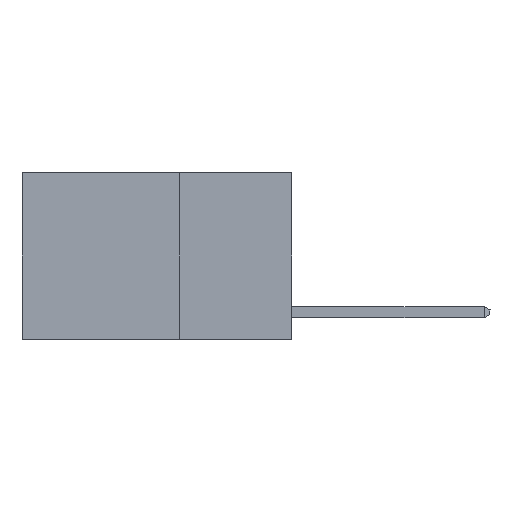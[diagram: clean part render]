
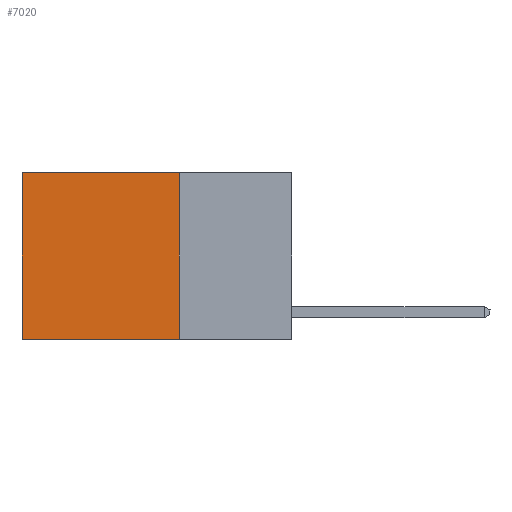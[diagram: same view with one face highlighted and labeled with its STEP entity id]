
A CAD part, left-side view. The second image highlights one B-rep face of the part: STEP entity #7020.
In plain terms, the highlighted planar face has unit normal (-1, 0, 0).
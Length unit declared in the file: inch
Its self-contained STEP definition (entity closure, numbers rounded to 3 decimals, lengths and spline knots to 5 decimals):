
#259 = LINE ( 'NONE', #1123, #986 ) ;
#496 = ORIENTED_EDGE ( 'NONE', *, *, #2237, .F. ) ;
#986 = VECTOR ( 'NONE', #6802, 39.37008 ) ;
#1123 = CARTESIAN_POINT ( 'NONE',  ( 0.2625, 0.25, 0. ) ) ;
#2237 = EDGE_CURVE ( 'NONE', #4178, #6870, #11249, .T. ) ;
#2352 = ORIENTED_EDGE ( 'NONE', *, *, #13689, .F. ) ;
#3117 = EDGE_CURVE ( 'NONE', #12019, #12507, #4501, .T. ) ;
#3891 = CARTESIAN_POINT ( 'NONE',  ( 0.2625, 0.25, 0. ) ) ;
#4057 = CARTESIAN_POINT ( 'NONE',  ( 0.2625, 0.6, 0. ) ) ;
#4178 = VERTEX_POINT ( 'NONE', #6929 ) ;
#4297 = LINE ( 'NONE', #11072, #13867 ) ;
#4501 = LINE ( 'NONE', #6597, #10852 ) ;
#5128 = PLANE ( 'NONE',  #10225 ) ;
#5749 = ORIENTED_EDGE ( 'NONE', *, *, #3117, .T. ) ;
#6220 = DIRECTION ( 'NONE',  ( 1., 0., 0. ) ) ;
#6271 = DIRECTION ( 'NONE',  ( 0., 0., -1. ) ) ;
#6578 = CARTESIAN_POINT ( 'NONE',  ( 0.2625, 0.25, 0. ) ) ;
#6597 = CARTESIAN_POINT ( 'NONE',  ( 0.2625, 0.6, 0. ) ) ;
#6802 = DIRECTION ( 'NONE',  ( 0., 1., 0. ) ) ;
#6870 = VERTEX_POINT ( 'NONE', #11126 ) ;
#6929 = CARTESIAN_POINT ( 'NONE',  ( 0.2625, 0.25, 0. ) ) ;
#7020 = ADVANCED_FACE ( 'NONE', ( #13658 ), #5128, .F. ) ;
#7344 = EDGE_LOOP ( 'NONE', ( #5749, #2352, #496, #9661 ) ) ;
#7915 = EDGE_CURVE ( 'NONE', #4178, #12019, #259, .T. ) ;
#8745 = DIRECTION ( 'NONE',  ( 0., 1., 0. ) ) ;
#9661 = ORIENTED_EDGE ( 'NONE', *, *, #7915, .T. ) ;
#10225 = AXIS2_PLACEMENT_3D ( 'NONE', #6578, #6220, #6271 ) ;
#10852 = VECTOR ( 'NONE', #14665, 39.37008 ) ;
#11072 = CARTESIAN_POINT ( 'NONE',  ( 0.2625, 0.25, -0.37 ) ) ;
#11126 = CARTESIAN_POINT ( 'NONE',  ( 0.2625, 0.25, -0.37 ) ) ;
#11249 = LINE ( 'NONE', #3891, #12124 ) ;
#12019 = VERTEX_POINT ( 'NONE', #4057 ) ;
#12124 = VECTOR ( 'NONE', #14280, 39.37008 ) ;
#12507 = VERTEX_POINT ( 'NONE', #13739 ) ;
#13658 = FACE_OUTER_BOUND ( 'NONE', #7344, .T. ) ;
#13689 = EDGE_CURVE ( 'NONE', #6870, #12507, #4297, .T. ) ;
#13739 = CARTESIAN_POINT ( 'NONE',  ( 0.2625, 0.6, -0.37 ) ) ;
#13867 = VECTOR ( 'NONE', #8745, 39.37008 ) ;
#14280 = DIRECTION ( 'NONE',  ( 0., 0., -1. ) ) ;
#14665 = DIRECTION ( 'NONE',  ( 0., 0., -1. ) ) ;
